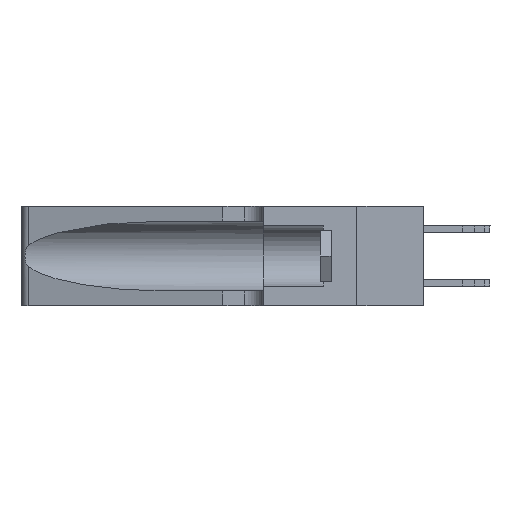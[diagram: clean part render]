
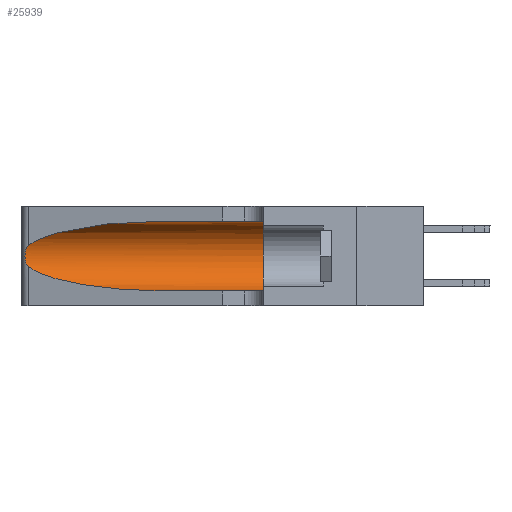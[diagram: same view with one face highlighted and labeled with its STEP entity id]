
A CAD part, left-side view. The second image highlights one B-rep face of the part: STEP entity #25939.
In plain terms, the highlighted cylindrical face has radius 3.308 mm (diameter 6.617 mm), a partial arc.
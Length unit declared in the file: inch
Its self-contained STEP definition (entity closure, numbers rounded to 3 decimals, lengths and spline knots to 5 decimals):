
#1181 = ORIENTED_EDGE ( 'NONE', *, *, #30690, .T. ) ;
#1199 = CYLINDRICAL_SURFACE ( 'NONE', #3034, 0.13025 ) ;
#3034 = AXIS2_PLACEMENT_3D ( 'NONE', #31819, #26153, #9480 ) ;
#4219 = CARTESIAN_POINT ( 'NONE',  ( 0.25487, 1.22718, 0.14631 ) ) ;
#4326 = CARTESIAN_POINT ( 'NONE',  ( 0.25487, 1.22718, 0.14631 ) ) ;
#4333 = CARTESIAN_POINT ( 'NONE',  ( 0.2373, 1.15595, 0.08982 ) ) ;
#4595 = CARTESIAN_POINT ( 'NONE',  ( 0.1305, 0.72297, 0.31525 ) ) ;
#4634 = CARTESIAN_POINT ( 'NONE',  ( 0.1305, 0.35, 0.31525 ) ) ;
#5635 = CARTESIAN_POINT ( 'NONE',  ( 0.1305, 1.61858, 0.05475 ) ) ;
#5958 = VERTEX_POINT ( 'NONE', #4634 ) ;
#6614 = LINE ( 'NONE', #20127, #8408 ) ;
#7068 = CIRCLE ( 'NONE', #27637, 0.13025 ) ;
#7252 = CARTESIAN_POINT ( 'NONE',  ( 0.26017, 1.23833, 0.17102 ) ) ;
#8106 = B_SPLINE_CURVE_WITH_KNOTS ( 'NONE', 3,
 ( #29949, #18392, #30076, #18768, #12782, #35730, #13280, #32927, #7252, #21451, #16006, #27233, #32538, #4326 ),
 .UNSPECIFIED., .F., .F.,
 ( 4, 2, 2, 2, 2, 2, 4 ),
 ( 0., 0.00027, 0.00053, 0.00107, 0.0016, 0.00187, 0.00214 ),
 .UNSPECIFIED. ) ;
#8408 = VECTOR ( 'NONE', #29720, 39.37008 ) ;
#8956 = EDGE_CURVE ( 'NONE', #5958, #27571, #7068, .T. ) ;
#9480 = DIRECTION ( 'NONE',  ( 0., 0., -1. ) ) ;
#10975 = VERTEX_POINT ( 'NONE', #15133 ) ;
#11183 = DIRECTION ( 'NONE',  ( 0., -1., 0. ) ) ;
#12439 = CARTESIAN_POINT ( 'NONE',  ( 0.2373, 1.15595, 0.28018 ) ) ;
#12782 = CARTESIAN_POINT ( 'NONE',  ( 0.25854, 1.2359, 0.20912 ) ) ;
#13280 = CARTESIAN_POINT ( 'NONE',  ( 0.26075, 1.23896, 0.19203 ) ) ;
#13514 =( BOUNDED_CURVE ( )  B_SPLINE_CURVE ( 3, ( #4219, #4333, #32424, #24173 ),
 .UNSPECIFIED., .F., .T. ) 
 B_SPLINE_CURVE_WITH_KNOTS ( ( 4, 4 ),
 ( 3.44316, 4.71239 ),
 .UNSPECIFIED. ) 
 CURVE ( )  GEOMETRIC_REPRESENTATION_ITEM ( )  RATIONAL_B_SPLINE_CURVE ( ( 1., 0.87, 0.87, 1. ) ) 
 REPRESENTATION_ITEM ( '' )  );
#14011 = DIRECTION ( 'NONE',  ( 0., 0., 1. ) ) ;
#14626 =( BOUNDED_CURVE ( )  B_SPLINE_CURVE ( 3, ( #4595, #24180, #12439, #15270 ),
 .UNSPECIFIED., .F., .F. ) 
 B_SPLINE_CURVE_WITH_KNOTS ( ( 4, 4 ),
 ( 1.5708, 2.84003 ),
 .UNSPECIFIED. ) 
 CURVE ( )  GEOMETRIC_REPRESENTATION_ITEM ( )  RATIONAL_B_SPLINE_CURVE ( ( 1., 0.87, 0.87, 1. ) ) 
 REPRESENTATION_ITEM ( '' )  );
#15133 = CARTESIAN_POINT ( 'NONE',  ( 0.25487, 1.22718, 0.22369 ) ) ;
#15270 = CARTESIAN_POINT ( 'NONE',  ( 0.25487, 1.22718, 0.22369 ) ) ;
#15297 = VERTEX_POINT ( 'NONE', #26226 ) ;
#15793 = CARTESIAN_POINT ( 'NONE',  ( 0.1305, 0.35, 0.05475 ) ) ;
#16006 = CARTESIAN_POINT ( 'NONE',  ( 0.25789, 1.23486, 0.15765 ) ) ;
#18392 = CARTESIAN_POINT ( 'NONE',  ( 0.25555, 1.22994, 0.2215 ) ) ;
#18768 = CARTESIAN_POINT ( 'NONE',  ( 0.25787, 1.23484, 0.2124 ) ) ;
#20056 = DIRECTION ( 'NONE',  ( 0., 1., 0. ) ) ;
#20127 = CARTESIAN_POINT ( 'NONE',  ( 0.1305, 1.61858, 0.31525 ) ) ;
#20756 = VECTOR ( 'NONE', #11183, 39.37008 ) ;
#21055 = EDGE_LOOP ( 'NONE', ( #1181, #35105, #30183, #21524, #35721, #29882 ) ) ;
#21451 = CARTESIAN_POINT ( 'NONE',  ( 0.25856, 1.23593, 0.16098 ) ) ;
#21524 = ORIENTED_EDGE ( 'NONE', *, *, #33956, .T. ) ;
#21734 = EDGE_CURVE ( 'NONE', #15297, #36224, #13514, .T. ) ;
#24173 = CARTESIAN_POINT ( 'NONE',  ( 0.1305, 0.72297, 0.05475 ) ) ;
#24180 = CARTESIAN_POINT ( 'NONE',  ( 0.18966, 0.96281, 0.31525 ) ) ;
#25083 = VERTEX_POINT ( 'NONE', #28294 ) ;
#25481 = CARTESIAN_POINT ( 'NONE',  ( 0.1305, 0.35, 0.185 ) ) ;
#25939 = ADVANCED_FACE ( 'NONE', ( #28850 ), #1199, .F. ) ;
#26153 = DIRECTION ( 'NONE',  ( 0., -1., 0. ) ) ;
#26226 = CARTESIAN_POINT ( 'NONE',  ( 0.25487, 1.22718, 0.14631 ) ) ;
#27233 = CARTESIAN_POINT ( 'NONE',  ( 0.25639, 1.23186, 0.15144 ) ) ;
#27571 = VERTEX_POINT ( 'NONE', #15793 ) ;
#27637 = AXIS2_PLACEMENT_3D ( 'NONE', #25481, #20056, #14011 ) ;
#28294 = CARTESIAN_POINT ( 'NONE',  ( 0.1305, 0.72297, 0.31525 ) ) ;
#28850 = FACE_OUTER_BOUND ( 'NONE', #21055, .T. ) ;
#29514 = CARTESIAN_POINT ( 'NONE',  ( 0.1305, 0.72297, 0.05475 ) ) ;
#29720 = DIRECTION ( 'NONE',  ( 0., -1., 0. ) ) ;
#29882 = ORIENTED_EDGE ( 'NONE', *, *, #34922, .F. ) ;
#29949 = CARTESIAN_POINT ( 'NONE',  ( 0.25487, 1.22718, 0.22369 ) ) ;
#30076 = CARTESIAN_POINT ( 'NONE',  ( 0.25639, 1.23184, 0.21858 ) ) ;
#30183 = ORIENTED_EDGE ( 'NONE', *, *, #21734, .T. ) ;
#30690 = EDGE_CURVE ( 'NONE', #25083, #10975, #14626, .T. ) ;
#31819 = CARTESIAN_POINT ( 'NONE',  ( 0.1305, 1.61858, 0.185 ) ) ;
#31980 = EDGE_CURVE ( 'NONE', #10975, #15297, #8106, .T. ) ;
#32424 = CARTESIAN_POINT ( 'NONE',  ( 0.18966, 0.96281, 0.05475 ) ) ;
#32538 = CARTESIAN_POINT ( 'NONE',  ( 0.25555, 1.22993, 0.14849 ) ) ;
#32927 = CARTESIAN_POINT ( 'NONE',  ( 0.26075, 1.23896, 0.178 ) ) ;
#33956 = EDGE_CURVE ( 'NONE', #36224, #27571, #34380, .T. ) ;
#34380 = LINE ( 'NONE', #5635, #20756 ) ;
#34922 = EDGE_CURVE ( 'NONE', #25083, #5958, #6614, .T. ) ;
#35105 = ORIENTED_EDGE ( 'NONE', *, *, #31980, .T. ) ;
#35721 = ORIENTED_EDGE ( 'NONE', *, *, #8956, .F. ) ;
#35730 = CARTESIAN_POINT ( 'NONE',  ( 0.26018, 1.23835, 0.19895 ) ) ;
#36224 = VERTEX_POINT ( 'NONE', #29514 ) ;
